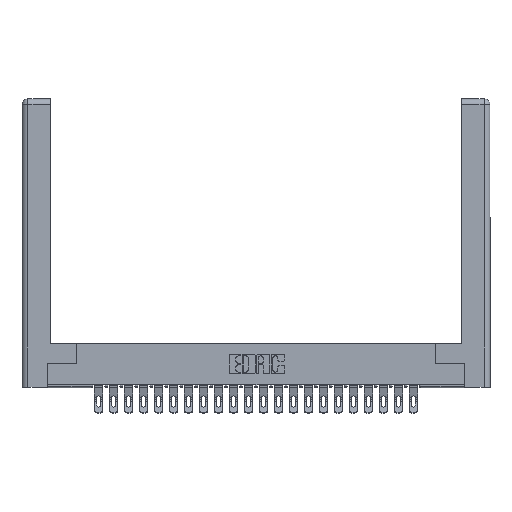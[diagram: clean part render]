
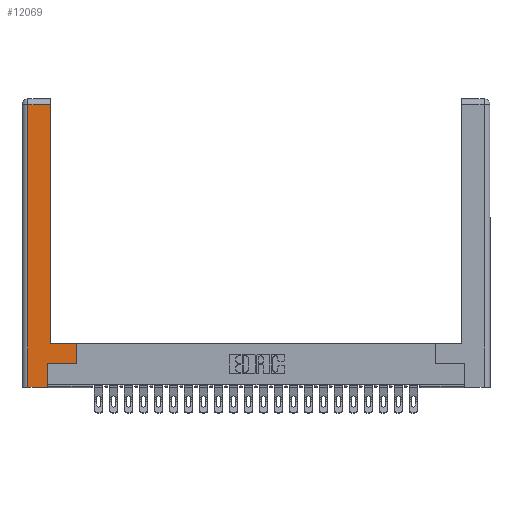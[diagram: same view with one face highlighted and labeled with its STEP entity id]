
A CAD part, top view. The second image highlights one B-rep face of the part: STEP entity #12069.
In plain terms, the highlighted planar face has unit normal (0, 0, 1).
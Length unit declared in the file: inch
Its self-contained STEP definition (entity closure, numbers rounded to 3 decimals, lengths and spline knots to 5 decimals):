
#475 = EDGE_CURVE ( 'NONE', #29088, #7216, #12807, .T. ) ;
#765 = AXIS2_PLACEMENT_3D ( 'NONE', #5846, #7940, #1255 ) ;
#1004 = CARTESIAN_POINT ( 'NONE',  ( 0.265, 0., 0. ) ) ;
#1255 = DIRECTION ( 'NONE',  ( -1., 0., 0. ) ) ;
#1315 = DIRECTION ( 'NONE',  ( -1., 0., 0. ) ) ;
#2073 = CARTESIAN_POINT ( 'NONE',  ( 0.295, 2.94, 0. ) ) ;
#3466 = VERTEX_POINT ( 'NONE', #10444 ) ;
#3572 = VERTEX_POINT ( 'NONE', #20096 ) ;
#4059 = LINE ( 'NONE', #25409, #19743 ) ;
#4090 = VERTEX_POINT ( 'NONE', #16844 ) ;
#4240 = EDGE_CURVE ( 'NONE', #7216, #9120, #25764, .T. ) ;
#4282 = EDGE_CURVE ( 'NONE', #3572, #3466, #24319, .T. ) ;
#5104 = LINE ( 'NONE', #21938, #19709 ) ;
#5122 = CARTESIAN_POINT ( 'NONE',  ( 0.295, 0.45, 0. ) ) ;
#5651 = ORIENTED_EDGE ( 'NONE', *, *, #25716, .T. ) ;
#5694 = CARTESIAN_POINT ( 'NONE',  ( 0.0615, 2.94, 0. ) ) ;
#5846 = CARTESIAN_POINT ( 'NONE',  ( 0., 0., 0. ) ) ;
#5851 = CARTESIAN_POINT ( 'NONE',  ( 0.565, 0.45, 0. ) ) ;
#6133 = VECTOR ( 'NONE', #16225, 39.37008 ) ;
#6453 = ORIENTED_EDGE ( 'NONE', *, *, #6498, .T. ) ;
#6468 = DIRECTION ( 'NONE',  ( 1., 0., 0. ) ) ;
#6498 = EDGE_CURVE ( 'NONE', #25504, #19434, #4059, .T. ) ;
#6952 = CARTESIAN_POINT ( 'NONE',  ( 0.265, 0.245, 0. ) ) ;
#7216 = VERTEX_POINT ( 'NONE', #5122 ) ;
#7940 = DIRECTION ( 'NONE',  ( 0., 0., -1. ) ) ;
#8171 = ORIENTED_EDGE ( 'NONE', *, *, #14496, .T. ) ;
#9120 = VERTEX_POINT ( 'NONE', #2073 ) ;
#9748 = ORIENTED_EDGE ( 'NONE', *, *, #475, .T. ) ;
#9936 = ORIENTED_EDGE ( 'NONE', *, *, #20313, .T. ) ;
#10444 = CARTESIAN_POINT ( 'NONE',  ( 0.265, 0.245, 0. ) ) ;
#10452 = CARTESIAN_POINT ( 'NONE',  ( 0.295, 0.45, 0. ) ) ;
#11124 = CARTESIAN_POINT ( 'NONE',  ( 0.0615, 0., 0. ) ) ;
#11131 = VECTOR ( 'NONE', #25935, 39.37008 ) ;
#12069 = ADVANCED_FACE ( 'NONE', ( #19823 ), #24196, .F. ) ;
#12807 = LINE ( 'NONE', #10452, #19185 ) ;
#12937 = LINE ( 'NONE', #24617, #15428 ) ;
#13609 = CARTESIAN_POINT ( 'NONE',  ( 0.0615, 2.94, 0. ) ) ;
#14496 = EDGE_CURVE ( 'NONE', #4090, #29088, #5104, .T. ) ;
#14684 = VECTOR ( 'NONE', #29393, 39.37008 ) ;
#14967 = ORIENTED_EDGE ( 'NONE', *, *, #4240, .T. ) ;
#15242 = EDGE_CURVE ( 'NONE', #3466, #4090, #12937, .T. ) ;
#15428 = VECTOR ( 'NONE', #6468, 39.37008 ) ;
#16029 = LINE ( 'NONE', #5694, #25300 ) ;
#16225 = DIRECTION ( 'NONE',  ( 0., 1., 0. ) ) ;
#16844 = CARTESIAN_POINT ( 'NONE',  ( 0.565, 0.245, 0. ) ) ;
#18403 = ORIENTED_EDGE ( 'NONE', *, *, #15242, .T. ) ;
#19185 = VECTOR ( 'NONE', #21797, 39.37008 ) ;
#19322 = LINE ( 'NONE', #1004, #11131 ) ;
#19434 = VERTEX_POINT ( 'NONE', #11124 ) ;
#19709 = VECTOR ( 'NONE', #24249, 39.37008 ) ;
#19743 = VECTOR ( 'NONE', #21190, 39.37008 ) ;
#19823 = FACE_OUTER_BOUND ( 'NONE', #29001, .T. ) ;
#20096 = CARTESIAN_POINT ( 'NONE',  ( 0.265, 0., 0. ) ) ;
#20313 = EDGE_CURVE ( 'NONE', #9120, #25504, #16029, .T. ) ;
#21190 = DIRECTION ( 'NONE',  ( 0., -1., 0. ) ) ;
#21797 = DIRECTION ( 'NONE',  ( -1., 0., 0. ) ) ;
#21938 = CARTESIAN_POINT ( 'NONE',  ( 0.565, 0.45, 0. ) ) ;
#24196 = PLANE ( 'NONE',  #765 ) ;
#24249 = DIRECTION ( 'NONE',  ( 0., 1., 0. ) ) ;
#24319 = LINE ( 'NONE', #6952, #6133 ) ;
#24404 = CARTESIAN_POINT ( 'NONE',  ( 0.295, 3., 0. ) ) ;
#24617 = CARTESIAN_POINT ( 'NONE',  ( 0.565, 0.245, 0. ) ) ;
#25300 = VECTOR ( 'NONE', #1315, 39.37008 ) ;
#25409 = CARTESIAN_POINT ( 'NONE',  ( 0.0615, 0., 0. ) ) ;
#25504 = VERTEX_POINT ( 'NONE', #13609 ) ;
#25716 = EDGE_CURVE ( 'NONE', #19434, #3572, #19322, .T. ) ;
#25764 = LINE ( 'NONE', #24404, #14684 ) ;
#25935 = DIRECTION ( 'NONE',  ( 1., 0., 0. ) ) ;
#28909 = ORIENTED_EDGE ( 'NONE', *, *, #4282, .T. ) ;
#29001 = EDGE_LOOP ( 'NONE', ( #14967, #9936, #6453, #5651, #28909, #18403, #8171, #9748 ) ) ;
#29088 = VERTEX_POINT ( 'NONE', #5851 ) ;
#29393 = DIRECTION ( 'NONE',  ( 0., 1., 0. ) ) ;
